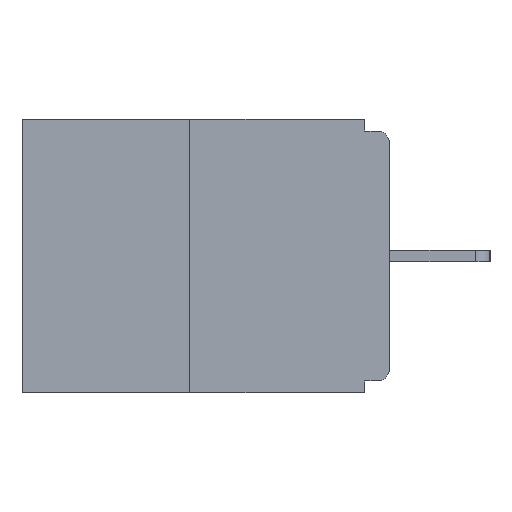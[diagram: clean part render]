
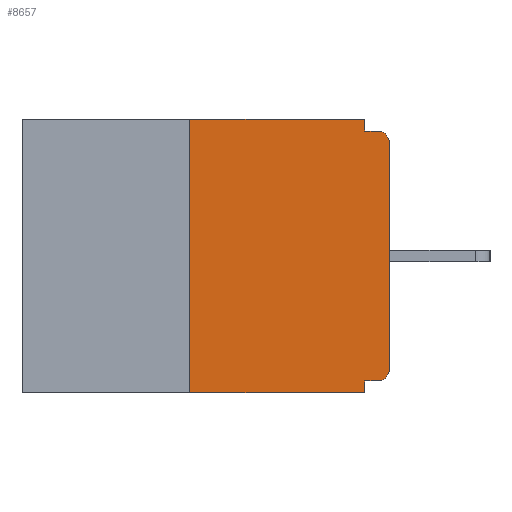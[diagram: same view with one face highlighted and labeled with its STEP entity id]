
A CAD part, left-side view. The second image highlights one B-rep face of the part: STEP entity #8657.
In plain terms, the highlighted planar face has unit normal (-1, 0, 0).
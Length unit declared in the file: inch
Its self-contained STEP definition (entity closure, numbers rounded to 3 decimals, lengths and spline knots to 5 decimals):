
#98 = ORIENTED_EDGE ( 'NONE', *, *, #3962, .T. ) ;
#128 = EDGE_LOOP ( 'NONE', ( #10574, #1149, #3644, #7576, #22297, #441, #2664, #98, #13733, #21917 ) ) ;
#191 = DIRECTION ( 'NONE',  ( -1., 0., 0. ) ) ;
#284 = DIRECTION ( 'NONE',  ( -1., 0., 0. ) ) ;
#382 = VECTOR ( 'NONE', #5650, 39.37008 ) ;
#441 = ORIENTED_EDGE ( 'NONE', *, *, #10413, .T. ) ;
#610 = VERTEX_POINT ( 'NONE', #17119 ) ;
#682 = CARTESIAN_POINT ( 'NONE',  ( 0., 0., 0. ) ) ;
#747 = VERTEX_POINT ( 'NONE', #2165 ) ;
#1149 = ORIENTED_EDGE ( 'NONE', *, *, #11227, .F. ) ;
#2165 = CARTESIAN_POINT ( 'NONE',  ( 0., 0.015, -0.015 ) ) ;
#2263 = CIRCLE ( 'NONE', #20957, 0.015 ) ;
#2664 = ORIENTED_EDGE ( 'NONE', *, *, #12589, .T. ) ;
#3235 = LINE ( 'NONE', #21348, #15062 ) ;
#3322 = CIRCLE ( 'NONE', #17640, 0.015 ) ;
#3644 = ORIENTED_EDGE ( 'NONE', *, *, #3661, .T. ) ;
#3661 = EDGE_CURVE ( 'NONE', #14131, #19183, #9480, .T. ) ;
#3936 = CARTESIAN_POINT ( 'NONE',  ( 0., 0.031, 0. ) ) ;
#3962 = EDGE_CURVE ( 'NONE', #6474, #747, #3322, .T. ) ;
#3983 = CARTESIAN_POINT ( 'NONE',  ( 0., 0.015, -0.328 ) ) ;
#4149 = DIRECTION ( 'NONE',  ( 0., 0., -1. ) ) ;
#4280 = EDGE_CURVE ( 'NONE', #19495, #5671, #10003, .T. ) ;
#4295 = CARTESIAN_POINT ( 'NONE',  ( 0., 0.46, -0.343 ) ) ;
#4603 = CARTESIAN_POINT ( 'NONE',  ( 0., 0.25, 0. ) ) ;
#5650 = DIRECTION ( 'NONE',  ( 0., 0., -1. ) ) ;
#5671 = VERTEX_POINT ( 'NONE', #7154 ) ;
#5940 = LINE ( 'NONE', #7657, #14404 ) ;
#5944 = DIRECTION ( 'NONE',  ( 0., 0., 1. ) ) ;
#6092 = CARTESIAN_POINT ( 'NONE',  ( 0., 0.46, 0. ) ) ;
#6474 = VERTEX_POINT ( 'NONE', #12835 ) ;
#6916 = CARTESIAN_POINT ( 'NONE',  ( 0., 0.031, -0.343 ) ) ;
#7106 = VERTEX_POINT ( 'NONE', #22547 ) ;
#7154 = CARTESIAN_POINT ( 'NONE',  ( 0., 0.031, 0. ) ) ;
#7259 = DIRECTION ( 'NONE',  ( 0., 0., -1. ) ) ;
#7576 = ORIENTED_EDGE ( 'NONE', *, *, #17957, .F. ) ;
#7657 = CARTESIAN_POINT ( 'NONE',  ( 0., 0.25, 0. ) ) ;
#8657 = ADVANCED_FACE ( 'NONE', ( #21843 ), #9548, .F. ) ;
#9256 = VECTOR ( 'NONE', #12548, 39.37008 ) ;
#9480 = LINE ( 'NONE', #4295, #20892 ) ;
#9537 = VECTOR ( 'NONE', #13807, 39.37008 ) ;
#9548 = PLANE ( 'NONE',  #20206 ) ;
#9561 = EDGE_CURVE ( 'NONE', #18882, #7106, #3235, .T. ) ;
#9666 = DIRECTION ( 'NONE',  ( 1., 0., 0. ) ) ;
#10003 = LINE ( 'NONE', #22173, #9537 ) ;
#10413 = EDGE_CURVE ( 'NONE', #18882, #18231, #2263, .T. ) ;
#10574 = ORIENTED_EDGE ( 'NONE', *, *, #4280, .F. ) ;
#10790 = DIRECTION ( 'NONE',  ( 0., 1., 0. ) ) ;
#11227 = EDGE_CURVE ( 'NONE', #14131, #19495, #5940, .T. ) ;
#11333 = DIRECTION ( 'NONE',  ( 0., -1., 0. ) ) ;
#11393 = CARTESIAN_POINT ( 'NONE',  ( 0., 0.25, -0.343 ) ) ;
#11913 = EDGE_CURVE ( 'NONE', #610, #747, #13933, .T. ) ;
#12233 = VECTOR ( 'NONE', #5944, 39.37008 ) ;
#12234 = LINE ( 'NONE', #3936, #12306 ) ;
#12306 = VECTOR ( 'NONE', #22669, 39.37008 ) ;
#12421 = CARTESIAN_POINT ( 'NONE',  ( 0., 0., -0.015 ) ) ;
#12548 = DIRECTION ( 'NONE',  ( 0., -1., 0. ) ) ;
#12566 = CARTESIAN_POINT ( 'NONE',  ( 0., 0.031, -0.343 ) ) ;
#12589 = EDGE_CURVE ( 'NONE', #18231, #6474, #16424, .T. ) ;
#12835 = CARTESIAN_POINT ( 'NONE',  ( 0., 0., -0.03 ) ) ;
#13733 = ORIENTED_EDGE ( 'NONE', *, *, #11913, .F. ) ;
#13807 = DIRECTION ( 'NONE',  ( 0., -1., 0. ) ) ;
#13933 = LINE ( 'NONE', #12421, #9256 ) ;
#13993 = EDGE_CURVE ( 'NONE', #5671, #610, #12234, .T. ) ;
#14131 = VERTEX_POINT ( 'NONE', #11393 ) ;
#14404 = VECTOR ( 'NONE', #14697, 39.37008 ) ;
#14697 = DIRECTION ( 'NONE',  ( 0., 0., 1. ) ) ;
#15062 = VECTOR ( 'NONE', #10790, 39.37008 ) ;
#15796 = LINE ( 'NONE', #6916, #382 ) ;
#16024 = CARTESIAN_POINT ( 'NONE',  ( 0., 0.015, -0.313 ) ) ;
#16424 = LINE ( 'NONE', #682, #12233 ) ;
#17119 = CARTESIAN_POINT ( 'NONE',  ( 0., 0.031, -0.015 ) ) ;
#17438 = DIRECTION ( 'NONE',  ( 0., 0., -1. ) ) ;
#17538 = CARTESIAN_POINT ( 'NONE',  ( 0., 0.015, -0.03 ) ) ;
#17640 = AXIS2_PLACEMENT_3D ( 'NONE', #17538, #191, #17438 ) ;
#17957 = EDGE_CURVE ( 'NONE', #7106, #19183, #15796, .T. ) ;
#18231 = VERTEX_POINT ( 'NONE', #18529 ) ;
#18529 = CARTESIAN_POINT ( 'NONE',  ( 0., 0., -0.313 ) ) ;
#18882 = VERTEX_POINT ( 'NONE', #3983 ) ;
#19183 = VERTEX_POINT ( 'NONE', #12566 ) ;
#19495 = VERTEX_POINT ( 'NONE', #4603 ) ;
#20206 = AXIS2_PLACEMENT_3D ( 'NONE', #6092, #9666, #4149 ) ;
#20892 = VECTOR ( 'NONE', #11333, 39.37008 ) ;
#20957 = AXIS2_PLACEMENT_3D ( 'NONE', #16024, #284, #7259 ) ;
#21348 = CARTESIAN_POINT ( 'NONE',  ( 0., 0., -0.328 ) ) ;
#21843 = FACE_OUTER_BOUND ( 'NONE', #128, .T. ) ;
#21917 = ORIENTED_EDGE ( 'NONE', *, *, #13993, .F. ) ;
#22173 = CARTESIAN_POINT ( 'NONE',  ( 0., 0.46, 0. ) ) ;
#22297 = ORIENTED_EDGE ( 'NONE', *, *, #9561, .F. ) ;
#22547 = CARTESIAN_POINT ( 'NONE',  ( 0., 0.031, -0.328 ) ) ;
#22669 = DIRECTION ( 'NONE',  ( 0., 0., -1. ) ) ;
